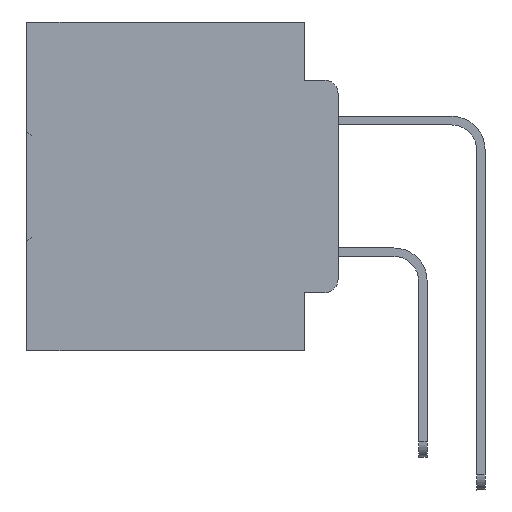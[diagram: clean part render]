
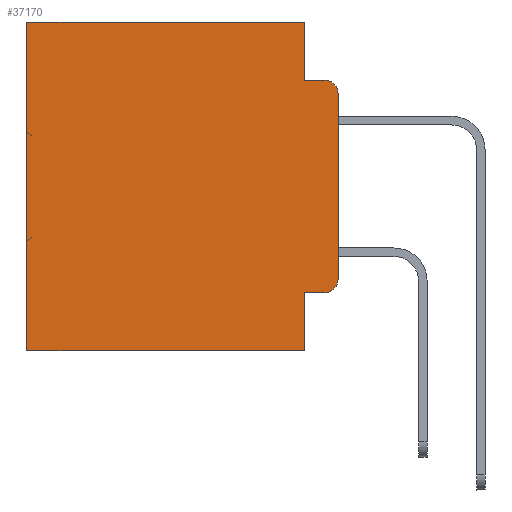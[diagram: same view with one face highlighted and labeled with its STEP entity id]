
A CAD part, left-side view. The second image highlights one B-rep face of the part: STEP entity #37170.
In plain terms, the highlighted planar face has unit normal (-1, 0, 0).
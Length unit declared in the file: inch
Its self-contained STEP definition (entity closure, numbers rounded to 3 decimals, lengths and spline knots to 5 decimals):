
#370 = DIRECTION ( 'NONE',  ( 0., 0., -1. ) ) ;
#516 = CARTESIAN_POINT ( 'NONE',  ( 0.298, 0.473, 0. ) ) ;
#1609 = DIRECTION ( 'NONE',  ( 1., 0., 0. ) ) ;
#1814 = PLANE ( 'NONE',  #7633 ) ;
#2286 = VECTOR ( 'NONE', #35500, 39.37008 ) ;
#3510 = CARTESIAN_POINT ( 'NONE',  ( 0.298, 0.473, 0. ) ) ;
#4204 = CARTESIAN_POINT ( 'NONE',  ( 0.298, 0.051, -0.4115 ) ) ;
#4684 = CARTESIAN_POINT ( 'NONE',  ( 0.298, 0., 0. ) ) ;
#5579 = EDGE_CURVE ( 'NONE', #11484, #15540, #9331, .T. ) ;
#5649 = CIRCLE ( 'NONE', #8062, 0.02 ) ;
#6079 = CARTESIAN_POINT ( 'NONE',  ( 0.298, 0.051, -0.0885 ) ) ;
#6171 = CARTESIAN_POINT ( 'NONE',  ( 0.298, 0., 0. ) ) ;
#6258 = DIRECTION ( 'NONE',  ( 0., -1., 0. ) ) ;
#6488 = ORIENTED_EDGE ( 'NONE', *, *, #30564, .F. ) ;
#6777 = CIRCLE ( 'NONE', #25076, 0.02 ) ;
#6847 = VECTOR ( 'NONE', #14074, 39.37008 ) ;
#6967 = CARTESIAN_POINT ( 'NONE',  ( 0.298, 0.02, -0.4115 ) ) ;
#7211 = VERTEX_POINT ( 'NONE', #6967 ) ;
#7311 = DIRECTION ( 'NONE',  ( 0., 0., -1. ) ) ;
#7536 = DIRECTION ( 'NONE',  ( 0., 0., -1. ) ) ;
#7633 = AXIS2_PLACEMENT_3D ( 'NONE', #4684, #1609, #7536 ) ;
#8062 = AXIS2_PLACEMENT_3D ( 'NONE', #30521, #27076, #18667 ) ;
#8202 = VECTOR ( 'NONE', #12654, 39.37008 ) ;
#9331 = LINE ( 'NONE', #34984, #21271 ) ;
#9469 = LINE ( 'NONE', #516, #2286 ) ;
#9883 = CARTESIAN_POINT ( 'NONE',  ( 0.298, 0.051, -0.5 ) ) ;
#10323 = CARTESIAN_POINT ( 'NONE',  ( 0.298, 0.051, -0.0885 ) ) ;
#10615 = LINE ( 'NONE', #25149, #6847 ) ;
#10984 = LINE ( 'NONE', #13872, #19955 ) ;
#11484 = VERTEX_POINT ( 'NONE', #12222 ) ;
#11874 = EDGE_CURVE ( 'NONE', #20620, #24604, #20026, .T. ) ;
#12222 = CARTESIAN_POINT ( 'NONE',  ( 0.298, 0., -0.1085 ) ) ;
#12408 = VECTOR ( 'NONE', #7311, 39.37008 ) ;
#12654 = DIRECTION ( 'NONE',  ( 0., 1., 0. ) ) ;
#13342 = EDGE_CURVE ( 'NONE', #7211, #15540, #5649, .T. ) ;
#13820 = DIRECTION ( 'NONE',  ( 0., -1., 0. ) ) ;
#13872 = CARTESIAN_POINT ( 'NONE',  ( 0.298, 0., -0.5 ) ) ;
#14074 = DIRECTION ( 'NONE',  ( 0., 0., -1. ) ) ;
#15349 = CARTESIAN_POINT ( 'NONE',  ( 0.298, 0.473, -0.5 ) ) ;
#15540 = VERTEX_POINT ( 'NONE', #23147 ) ;
#16514 = VERTEX_POINT ( 'NONE', #23050 ) ;
#17114 = CARTESIAN_POINT ( 'NONE',  ( 0.298, 0.02, -0.0885 ) ) ;
#17261 = EDGE_CURVE ( 'NONE', #27066, #7211, #28143, .T. ) ;
#17555 = ORIENTED_EDGE ( 'NONE', *, *, #22728, .T. ) ;
#18213 = EDGE_CURVE ( 'NONE', #24042, #37529, #10984, .T. ) ;
#18385 = LINE ( 'NONE', #6171, #8202 ) ;
#18667 = DIRECTION ( 'NONE',  ( 0., 0., -1. ) ) ;
#19186 = ORIENTED_EDGE ( 'NONE', *, *, #33672, .F. ) ;
#19955 = VECTOR ( 'NONE', #25516, 39.37008 ) ;
#20026 = LINE ( 'NONE', #6079, #33757 ) ;
#20375 = EDGE_LOOP ( 'NONE', ( #32119, #23366, #33461, #19186, #26670, #17555, #29105, #6488, #24517, #21759 ) ) ;
#20620 = VERTEX_POINT ( 'NONE', #10323 ) ;
#21150 = FACE_OUTER_BOUND ( 'NONE', #20375, .T. ) ;
#21271 = VECTOR ( 'NONE', #370, 39.37008 ) ;
#21759 = ORIENTED_EDGE ( 'NONE', *, *, #13342, .T. ) ;
#21836 = CARTESIAN_POINT ( 'NONE',  ( 0.298, 0.051, -0.4115 ) ) ;
#22728 = EDGE_CURVE ( 'NONE', #35638, #37529, #9469, .T. ) ;
#23050 = CARTESIAN_POINT ( 'NONE',  ( 0.298, 0.051, 0. ) ) ;
#23147 = CARTESIAN_POINT ( 'NONE',  ( 0.298, 0., -0.3915 ) ) ;
#23366 = ORIENTED_EDGE ( 'NONE', *, *, #26217, .T. ) ;
#24042 = VERTEX_POINT ( 'NONE', #9883 ) ;
#24517 = ORIENTED_EDGE ( 'NONE', *, *, #17261, .T. ) ;
#24604 = VERTEX_POINT ( 'NONE', #17114 ) ;
#25076 = AXIS2_PLACEMENT_3D ( 'NONE', #36019, #30645, #33156 ) ;
#25149 = CARTESIAN_POINT ( 'NONE',  ( 0.298, 0.051, 0. ) ) ;
#25516 = DIRECTION ( 'NONE',  ( 0., 1., 0. ) ) ;
#26217 = EDGE_CURVE ( 'NONE', #11484, #24604, #6777, .T. ) ;
#26670 = ORIENTED_EDGE ( 'NONE', *, *, #36188, .T. ) ;
#27066 = VERTEX_POINT ( 'NONE', #4204 ) ;
#27076 = DIRECTION ( 'NONE',  ( -1., 0., 0. ) ) ;
#27949 = CARTESIAN_POINT ( 'NONE',  ( 0.298, 0.051, 0. ) ) ;
#28143 = LINE ( 'NONE', #21836, #37009 ) ;
#29105 = ORIENTED_EDGE ( 'NONE', *, *, #18213, .F. ) ;
#30521 = CARTESIAN_POINT ( 'NONE',  ( 0.298, 0.02, -0.3915 ) ) ;
#30564 = EDGE_CURVE ( 'NONE', #27066, #24042, #33906, .T. ) ;
#30645 = DIRECTION ( 'NONE',  ( -1., 0., 0. ) ) ;
#32119 = ORIENTED_EDGE ( 'NONE', *, *, #5579, .F. ) ;
#33156 = DIRECTION ( 'NONE',  ( 0., 0., -1. ) ) ;
#33461 = ORIENTED_EDGE ( 'NONE', *, *, #11874, .F. ) ;
#33672 = EDGE_CURVE ( 'NONE', #16514, #20620, #10615, .T. ) ;
#33757 = VECTOR ( 'NONE', #6258, 39.37008 ) ;
#33906 = LINE ( 'NONE', #27949, #12408 ) ;
#34984 = CARTESIAN_POINT ( 'NONE',  ( 0.298, 0., 0. ) ) ;
#35500 = DIRECTION ( 'NONE',  ( 0., 0., -1. ) ) ;
#35638 = VERTEX_POINT ( 'NONE', #3510 ) ;
#36019 = CARTESIAN_POINT ( 'NONE',  ( 0.298, 0.02, -0.1085 ) ) ;
#36188 = EDGE_CURVE ( 'NONE', #16514, #35638, #18385, .T. ) ;
#37009 = VECTOR ( 'NONE', #13820, 39.37008 ) ;
#37170 = ADVANCED_FACE ( 'NONE', ( #21150 ), #1814, .F. ) ;
#37529 = VERTEX_POINT ( 'NONE', #15349 ) ;
